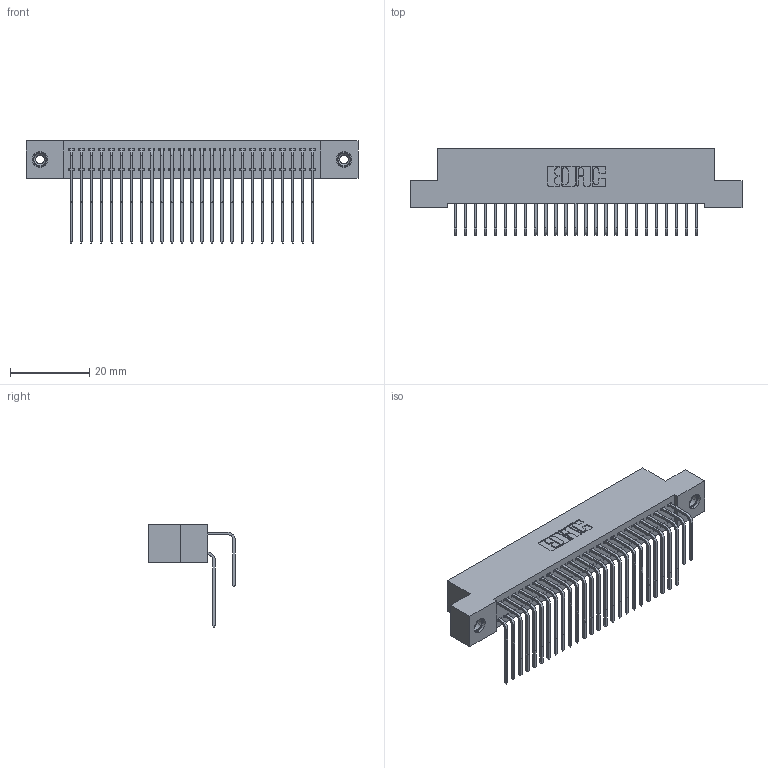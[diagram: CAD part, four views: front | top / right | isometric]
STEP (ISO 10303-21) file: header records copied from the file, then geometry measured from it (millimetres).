
FILE_DESCRIPTION (( 'STEP AP203' ), '1' );
FILE_NAME ('342-050-558-208.STEP', '2019-10-03T00:05:28', ( '' ), ( '' ), 'SwSTEP 2.0', 'SolidWorks 2016', '' );
FILE_SCHEMA (( 'CONFIG_CONTROL_DESIGN' ));
Length unit declared in the file: inch
Products named in the file (5): 342-050-558-208; 342 Part_TI; 345-292-001_558 559 Tail - 1; 345-292-001_558 Tail - 2; 345-250-001_345-250-003-102
Assembly tree (53 placements, depth 2):
  342-050-558-208
    342 Part_TI
    345-292-001_558 559 Tail - 1  x25
    345-292-001_558 Tail - 2  x25
    345-250-001_345-250-003-102  x2
Bounding box: 83.82 x 21.91 x 25.78 mm (x, y, z)
Volume: 7733.5 mm3; surface area: 13484.4 mm2
Topology: 53 solids, 53 shells, 2870 faces, 8485 edges, 5582 vertices
Faces by surface type: plane 1998, cylinder 856, cone 12, torus 4
Entity records: 21120 total; most frequent: CARTESIAN_POINT 3552, ORIENTED_EDGE 3430, DIRECTION 3077, EDGE_CURVE 1715, LINE 1527, VECTOR 1527, VERTEX_POINT 1136, AXIS2_PLACEMENT_3D 775
